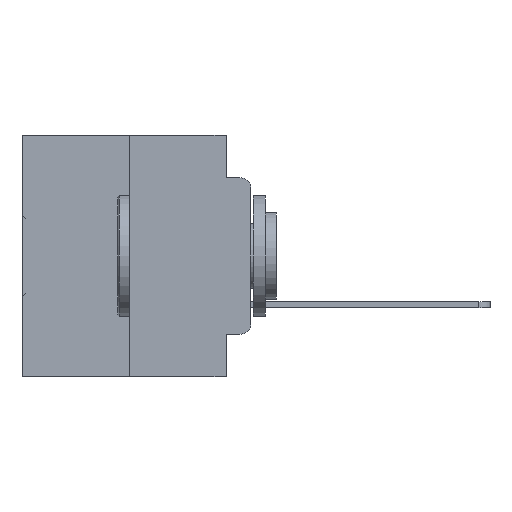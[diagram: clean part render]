
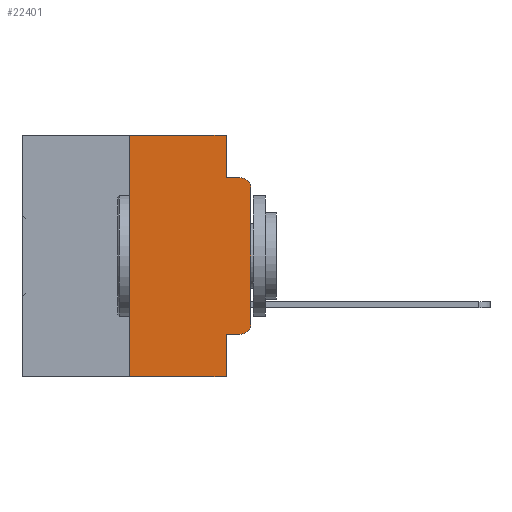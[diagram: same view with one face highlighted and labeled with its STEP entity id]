
A CAD part, left-side view. The second image highlights one B-rep face of the part: STEP entity #22401.
In plain terms, the highlighted planar face has unit normal (-1, 0, 0).
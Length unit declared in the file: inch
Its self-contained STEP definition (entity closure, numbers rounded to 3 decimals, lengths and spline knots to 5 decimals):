
#50 = ORIENTED_EDGE ( 'NONE', *, *, #9958, .F. ) ;
#571 = DIRECTION ( 'NONE',  ( 0., -1., 0. ) ) ;
#966 = CARTESIAN_POINT ( 'NONE',  ( 0., 0.473, 0. ) ) ;
#2053 = EDGE_CURVE ( 'NONE', #25368, #11943, #32383, .T. ) ;
#2209 = VECTOR ( 'NONE', #27073, 39.37008 ) ;
#2675 = ORIENTED_EDGE ( 'NONE', *, *, #6042, .F. ) ;
#3057 = ORIENTED_EDGE ( 'NONE', *, *, #13776, .T. ) ;
#3541 = CARTESIAN_POINT ( 'NONE',  ( 0., 0.02, -0.4115 ) ) ;
#3708 = VECTOR ( 'NONE', #17248, 39.37008 ) ;
#4057 = EDGE_CURVE ( 'NONE', #5542, #28889, #28474, .T. ) ;
#4395 = CARTESIAN_POINT ( 'NONE',  ( 0., 0.02, -0.0885 ) ) ;
#4663 = ORIENTED_EDGE ( 'NONE', *, *, #24408, .F. ) ;
#5331 = ORIENTED_EDGE ( 'NONE', *, *, #4057, .F. ) ;
#5542 = VERTEX_POINT ( 'NONE', #15101 ) ;
#5555 = ORIENTED_EDGE ( 'NONE', *, *, #8865, .T. ) ;
#5715 = DIRECTION ( 'NONE',  ( -1., 0., 0. ) ) ;
#5973 = ORIENTED_EDGE ( 'NONE', *, *, #11886, .T. ) ;
#6042 = EDGE_CURVE ( 'NONE', #30475, #23497, #20530, .T. ) ;
#6305 = CARTESIAN_POINT ( 'NONE',  ( 0., 0.25, 0. ) ) ;
#6392 = DIRECTION ( 'NONE',  ( 0., 0., -1. ) ) ;
#6393 = LINE ( 'NONE', #966, #33564 ) ;
#6679 = ORIENTED_EDGE ( 'NONE', *, *, #2053, .F. ) ;
#6940 = DIRECTION ( 'NONE',  ( 0., 0., 1. ) ) ;
#7159 = CARTESIAN_POINT ( 'NONE',  ( 0., 0.051, 0. ) ) ;
#7203 = ORIENTED_EDGE ( 'NONE', *, *, #33972, .T. ) ;
#7239 = ORIENTED_EDGE ( 'NONE', *, *, #32311, .T. ) ;
#7418 = LINE ( 'NONE', #15194, #15029 ) ;
#7485 = VECTOR ( 'NONE', #33379, 39.37008 ) ;
#8865 = EDGE_CURVE ( 'NONE', #5542, #11943, #34531, .T. ) ;
#9958 = EDGE_CURVE ( 'NONE', #23497, #21440, #7418, .T. ) ;
#10034 = CARTESIAN_POINT ( 'NONE',  ( 0., 0., -0.3915 ) ) ;
#10609 = CARTESIAN_POINT ( 'NONE',  ( 0., 0.25, 0. ) ) ;
#10610 = CARTESIAN_POINT ( 'NONE',  ( 0., 0.473, -0.5 ) ) ;
#11083 = DIRECTION ( 'NONE',  ( 1., 0., 0. ) ) ;
#11886 = EDGE_CURVE ( 'NONE', #32178, #21440, #30231, .T. ) ;
#11943 = VERTEX_POINT ( 'NONE', #14501 ) ;
#12669 = DIRECTION ( 'NONE',  ( 0., -1., 0. ) ) ;
#13776 = EDGE_CURVE ( 'NONE', #27279, #32178, #17606, .T. ) ;
#14501 = CARTESIAN_POINT ( 'NONE',  ( 0., 0.051, -0.5 ) ) ;
#15029 = VECTOR ( 'NONE', #571, 39.37008 ) ;
#15101 = CARTESIAN_POINT ( 'NONE',  ( 0., 0.25, -0.5 ) ) ;
#15175 = CARTESIAN_POINT ( 'NONE',  ( 0., 0.02, -0.3915 ) ) ;
#15194 = CARTESIAN_POINT ( 'NONE',  ( 0., 0.051, -0.0885 ) ) ;
#16349 = FACE_OUTER_BOUND ( 'NONE', #24446, .T. ) ;
#17148 = AXIS2_PLACEMENT_3D ( 'NONE', #34950, #11083, #29970 ) ;
#17248 = DIRECTION ( 'NONE',  ( 0., -1., 0. ) ) ;
#17606 = LINE ( 'NONE', #23590, #30106 ) ;
#17903 = DIRECTION ( 'NONE',  ( 0., 0., -1. ) ) ;
#19023 = CARTESIAN_POINT ( 'NONE',  ( 0., 0.051, 0. ) ) ;
#19257 = PLANE ( 'NONE',  #17148 ) ;
#19849 = AXIS2_PLACEMENT_3D ( 'NONE', #22411, #5715, #25128 ) ;
#20530 = LINE ( 'NONE', #23072, #34446 ) ;
#21440 = VERTEX_POINT ( 'NONE', #4395 ) ;
#22401 = ADVANCED_FACE ( 'NONE', ( #16349 ), #19257, .F. ) ;
#22411 = CARTESIAN_POINT ( 'NONE',  ( 0., 0.02, -0.1085 ) ) ;
#22832 = CARTESIAN_POINT ( 'NONE',  ( 0., 0., -0.1085 ) ) ;
#23072 = CARTESIAN_POINT ( 'NONE',  ( 0., 0.051, 0. ) ) ;
#23077 = CARTESIAN_POINT ( 'NONE',  ( 0., 0.051, -0.0885 ) ) ;
#23497 = VERTEX_POINT ( 'NONE', #23077 ) ;
#23590 = CARTESIAN_POINT ( 'NONE',  ( 0., 0., 0. ) ) ;
#24227 = DIRECTION ( 'NONE',  ( 0., -1., 0. ) ) ;
#24408 = EDGE_CURVE ( 'NONE', #28889, #30475, #6393, .T. ) ;
#24446 = EDGE_LOOP ( 'NONE', ( #3057, #5973, #50, #2675, #4663, #5331, #5555, #6679, #7203, #7239 ) ) ;
#25128 = DIRECTION ( 'NONE',  ( 0., 0., -1. ) ) ;
#25368 = VERTEX_POINT ( 'NONE', #29539 ) ;
#26944 = AXIS2_PLACEMENT_3D ( 'NONE', #15175, #33675, #17903 ) ;
#27073 = DIRECTION ( 'NONE',  ( 0., 0., -1. ) ) ;
#27279 = VERTEX_POINT ( 'NONE', #10034 ) ;
#28474 = LINE ( 'NONE', #6305, #7485 ) ;
#28889 = VERTEX_POINT ( 'NONE', #10609 ) ;
#29539 = CARTESIAN_POINT ( 'NONE',  ( 0., 0.051, -0.4115 ) ) ;
#29970 = DIRECTION ( 'NONE',  ( 0., 0., -1. ) ) ;
#30106 = VECTOR ( 'NONE', #6940, 39.37008 ) ;
#30231 = CIRCLE ( 'NONE', #19849, 0.02 ) ;
#30475 = VERTEX_POINT ( 'NONE', #7159 ) ;
#30791 = VERTEX_POINT ( 'NONE', #3541 ) ;
#32060 = LINE ( 'NONE', #33072, #3708 ) ;
#32178 = VERTEX_POINT ( 'NONE', #22832 ) ;
#32311 = EDGE_CURVE ( 'NONE', #30791, #27279, #35602, .T. ) ;
#32383 = LINE ( 'NONE', #19023, #2209 ) ;
#33072 = CARTESIAN_POINT ( 'NONE',  ( 0., 0.051, -0.4115 ) ) ;
#33379 = DIRECTION ( 'NONE',  ( 0., 0., 1. ) ) ;
#33564 = VECTOR ( 'NONE', #12669, 39.37008 ) ;
#33675 = DIRECTION ( 'NONE',  ( -1., 0., 0. ) ) ;
#33737 = VECTOR ( 'NONE', #24227, 39.37008 ) ;
#33972 = EDGE_CURVE ( 'NONE', #25368, #30791, #32060, .T. ) ;
#34446 = VECTOR ( 'NONE', #6392, 39.37008 ) ;
#34531 = LINE ( 'NONE', #10610, #33737 ) ;
#34950 = CARTESIAN_POINT ( 'NONE',  ( 0., 0.473, 0. ) ) ;
#35602 = CIRCLE ( 'NONE', #26944, 0.02 ) ;
